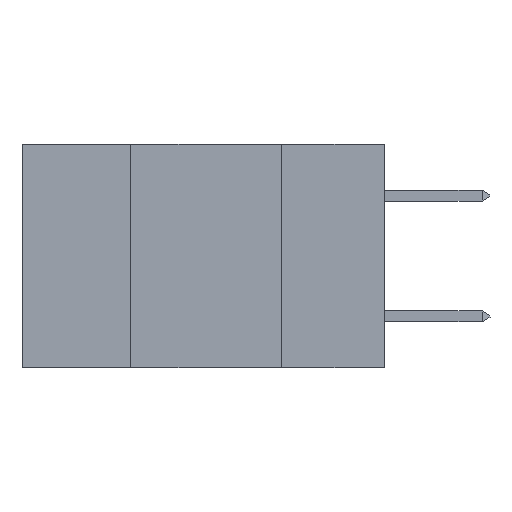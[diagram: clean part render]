
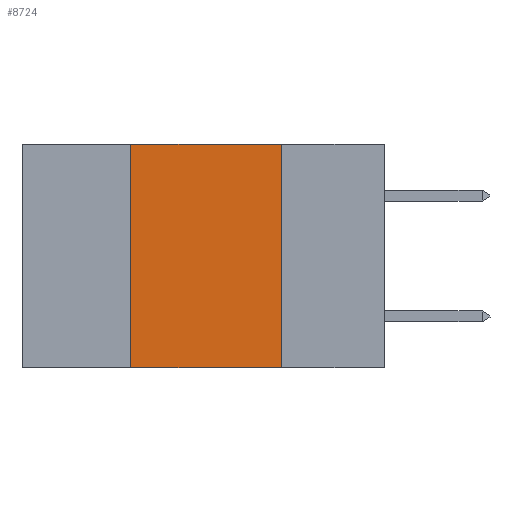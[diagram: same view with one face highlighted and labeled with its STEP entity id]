
A CAD part, left-side view. The second image highlights one B-rep face of the part: STEP entity #8724.
In plain terms, the highlighted planar face has unit normal (-1, 0, 0).
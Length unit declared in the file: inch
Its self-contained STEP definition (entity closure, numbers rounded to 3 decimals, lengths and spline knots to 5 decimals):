
#23 = CARTESIAN_POINT ( 'NONE',  ( 0., 0.42, 0. ) ) ;
#26 = DIRECTION ( 'NONE',  ( 0., 0., -1. ) ) ;
#356 = VERTEX_POINT ( 'NONE', #4199 ) ;
#428 = CARTESIAN_POINT ( 'NONE',  ( 0., 0.42, 0. ) ) ;
#653 = DIRECTION ( 'NONE',  ( 0., -1., 0. ) ) ;
#753 = DIRECTION ( 'NONE',  ( 0., 0., -1. ) ) ;
#1039 = EDGE_CURVE ( 'NONE', #16634, #356, #19230, .T. ) ;
#1184 = CARTESIAN_POINT ( 'NONE',  ( 0., 0.42, -0.37 ) ) ;
#1555 = CARTESIAN_POINT ( 'NONE',  ( 0., 0.17, 0. ) ) ;
#3373 = ORIENTED_EDGE ( 'NONE', *, *, #1039, .T. ) ;
#3470 = EDGE_CURVE ( 'NONE', #16370, #3700, #17618, .T. ) ;
#3700 = VERTEX_POINT ( 'NONE', #16483 ) ;
#4199 = CARTESIAN_POINT ( 'NONE',  ( 0., 0.17, -0.37 ) ) ;
#4225 = CARTESIAN_POINT ( 'NONE',  ( 0., 0.6, -0.37 ) ) ;
#4697 = ORIENTED_EDGE ( 'NONE', *, *, #3470, .F. ) ;
#4959 = EDGE_LOOP ( 'NONE', ( #8950, #4697, #8179, #3373 ) ) ;
#5338 = VECTOR ( 'NONE', #5698, 39.37008 ) ;
#5698 = DIRECTION ( 'NONE',  ( 0., -1., 0. ) ) ;
#5875 = VECTOR ( 'NONE', #9155, 39.37008 ) ;
#7406 = VECTOR ( 'NONE', #653, 39.37008 ) ;
#8179 = ORIENTED_EDGE ( 'NONE', *, *, #17516, .F. ) ;
#8724 = ADVANCED_FACE ( 'NONE', ( #10855 ), #17255, .F. ) ;
#8950 = ORIENTED_EDGE ( 'NONE', *, *, #15499, .F. ) ;
#9155 = DIRECTION ( 'NONE',  ( 0., 0., 1. ) ) ;
#9350 = AXIS2_PLACEMENT_3D ( 'NONE', #15742, #9810, #753 ) ;
#9810 = DIRECTION ( 'NONE',  ( 1., 0., 0. ) ) ;
#10201 = LINE ( 'NONE', #23, #5875 ) ;
#10855 = FACE_OUTER_BOUND ( 'NONE', #4959, .T. ) ;
#12997 = CARTESIAN_POINT ( 'NONE',  ( 0., 0.6, 0. ) ) ;
#13069 = VECTOR ( 'NONE', #26, 39.37008 ) ;
#15499 = EDGE_CURVE ( 'NONE', #3700, #356, #17064, .T. ) ;
#15742 = CARTESIAN_POINT ( 'NONE',  ( 0., 0.6, 0. ) ) ;
#16370 = VERTEX_POINT ( 'NONE', #428 ) ;
#16483 = CARTESIAN_POINT ( 'NONE',  ( 0., 0.17, 0. ) ) ;
#16634 = VERTEX_POINT ( 'NONE', #1184 ) ;
#17064 = LINE ( 'NONE', #1555, #13069 ) ;
#17255 = PLANE ( 'NONE',  #9350 ) ;
#17516 = EDGE_CURVE ( 'NONE', #16634, #16370, #10201, .T. ) ;
#17618 = LINE ( 'NONE', #12997, #5338 ) ;
#19230 = LINE ( 'NONE', #4225, #7406 ) ;
